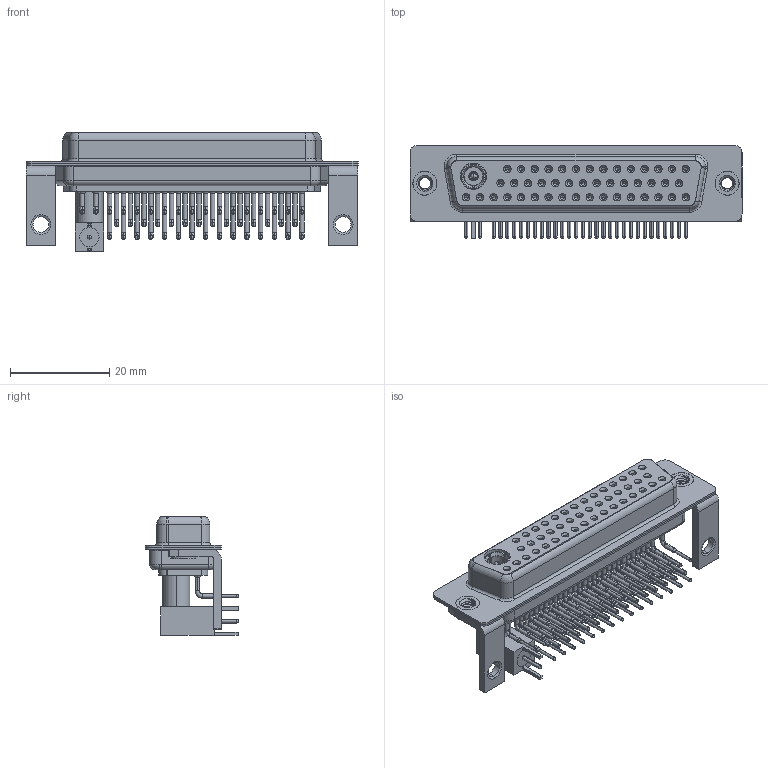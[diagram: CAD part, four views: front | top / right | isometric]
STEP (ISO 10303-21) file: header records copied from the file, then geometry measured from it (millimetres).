
FILE_DESCRIPTION (( 'STEP AP203' ), '1' );
FILE_NAME ('630-47W1240-5N4.STEP', '2022-06-10T08:13:15', ( '' ), ( '' ), 'SwSTEP 2.0', 'SolidWorks 2020', '' );
FILE_SCHEMA (( 'CONFIG_CONTROL_DESIGN' ));
Length unit declared in the file: millimetre
Products named in the file (16): RA Back Shell_50; Locking Collar; 630Combo Contact Row 1_50 Contacts; 630Combo Shell Front_50 Contacts; 630Combo Contact Row 2_50 Contacts; Insulator Pin_Straight PC Tail; 630Combo Shell Rear_50 Contacts; 630Combo Stabilizer Bracket_50 Contacts; 630Combo Contact Row 3; Insulator RA Pin; 630Combo Housing_47W1; Co-Ax Plug Assy_RA 50; Co-Ax Plug_RA 50; 630-47W1240-5N4; Pin_RA 50; 630Combo Threaded Rivet_3
Assembly tree (60 placements, depth 3):
  630-47W1240-5N4
    630Combo Housing_47W1
    630Combo Shell Front_50 Contacts
    630Combo Shell Rear_50 Contacts
    630Combo Threaded Rivet_3  x2
    630Combo Stabilizer Bracket_50 Contacts  x2
    Co-Ax Plug Assy_RA 50
      Co-Ax Plug_RA 50
      Insulator Pin_Straight PC Tail
      Pin_RA 50
      Locking Collar
      RA Back Shell_50
      Insulator RA Pin
    630Combo Contact Row 1_50 Contacts  x15
    630Combo Contact Row 2_50 Contacts  x14
    630Combo Contact Row 3  x17
Bounding box: 67 x 18.8 x 23.95 mm (x, y, z)
Volume: 7860.1 mm3; surface area: 17500 mm2
Topology: 59 solids, 59 shells, 2912 faces, 7374 edges, 4640 vertices
Faces by surface type: cylinder 1270, plane 841, cone 543, bspline 191, torus 63, sphere 4
Entity records: 37767 total; most frequent: CARTESIAN_POINT 7575, DIRECTION 6318, ORIENTED_EDGE 5230, AXIS2_PLACEMENT_3D 2637, EDGE_CURVE 2615, VERTEX_POINT 1670, CIRCLE 1450, EDGE_LOOP 1423
